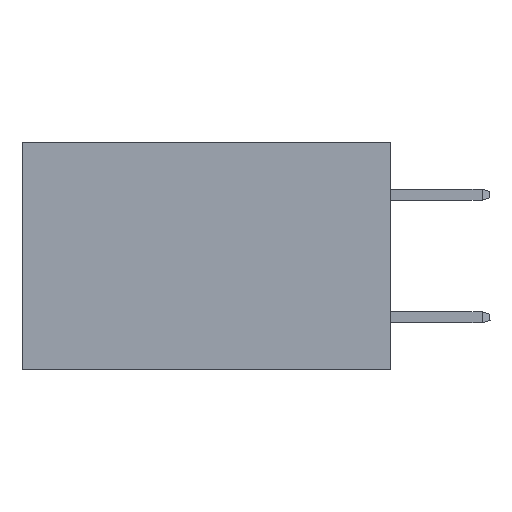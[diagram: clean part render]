
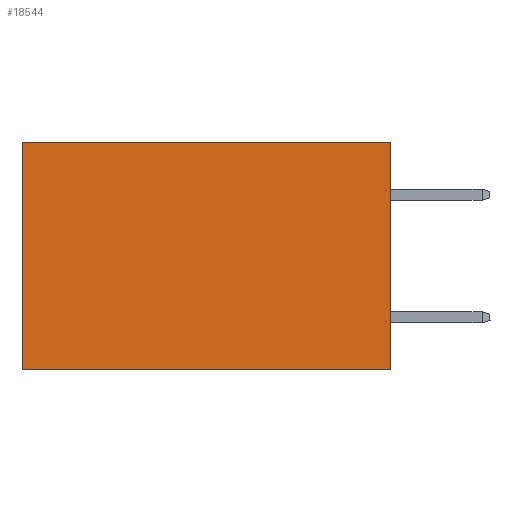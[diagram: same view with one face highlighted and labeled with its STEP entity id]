
A CAD part, left-side view. The second image highlights one B-rep face of the part: STEP entity #18544.
In plain terms, the highlighted planar face has unit normal (-1, 0, 0).
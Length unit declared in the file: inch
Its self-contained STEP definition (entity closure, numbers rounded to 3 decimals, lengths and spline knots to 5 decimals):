
#180 = VERTEX_POINT ( 'NONE', #13784 ) ;
#320 = VECTOR ( 'NONE', #20988, 39.37008 ) ;
#713 = EDGE_CURVE ( 'NONE', #6333, #1933, #5718, .T. ) ;
#1468 = DIRECTION ( 'NONE',  ( 1., 0., 0. ) ) ;
#1933 = VERTEX_POINT ( 'NONE', #5742 ) ;
#2020 = CARTESIAN_POINT ( 'NONE',  ( 0.2875, 0.6, 0. ) ) ;
#3017 = ORIENTED_EDGE ( 'NONE', *, *, #713, .F. ) ;
#4974 = CARTESIAN_POINT ( 'NONE',  ( 0.2875, 0., 0. ) ) ;
#5698 = ORIENTED_EDGE ( 'NONE', *, *, #15745, .T. ) ;
#5718 = LINE ( 'NONE', #10823, #8137 ) ;
#5742 = CARTESIAN_POINT ( 'NONE',  ( 0.2875, 0.6, -0.37 ) ) ;
#6333 = VERTEX_POINT ( 'NONE', #21174 ) ;
#7800 = DIRECTION ( 'NONE',  ( 0., 1., 0. ) ) ;
#8123 = PLANE ( 'NONE',  #17320 ) ;
#8137 = VECTOR ( 'NONE', #14182, 39.37008 ) ;
#8636 = LINE ( 'NONE', #2020, #320 ) ;
#10090 = CARTESIAN_POINT ( 'NONE',  ( 0.2875, 0., 0. ) ) ;
#10389 = ORIENTED_EDGE ( 'NONE', *, *, #11664, .T. ) ;
#10823 = CARTESIAN_POINT ( 'NONE',  ( 0.2875, 0., -0.37 ) ) ;
#11453 = VERTEX_POINT ( 'NONE', #13164 ) ;
#11664 = EDGE_CURVE ( 'NONE', #180, #1933, #8636, .T. ) ;
#11949 = DIRECTION ( 'NONE',  ( 0., 0., -1. ) ) ;
#12120 = EDGE_LOOP ( 'NONE', ( #10389, #3017, #12551, #5698 ) ) ;
#12551 = ORIENTED_EDGE ( 'NONE', *, *, #20283, .F. ) ;
#12940 = CARTESIAN_POINT ( 'NONE',  ( 0.2875, 0., 0. ) ) ;
#13164 = CARTESIAN_POINT ( 'NONE',  ( 0.2875, 0., 0. ) ) ;
#13668 = LINE ( 'NONE', #12940, #14219 ) ;
#13784 = CARTESIAN_POINT ( 'NONE',  ( 0.2875, 0.6, 0. ) ) ;
#14182 = DIRECTION ( 'NONE',  ( 0., 1., 0. ) ) ;
#14219 = VECTOR ( 'NONE', #7800, 39.37008 ) ;
#15089 = DIRECTION ( 'NONE',  ( 0., 0., -1. ) ) ;
#15745 = EDGE_CURVE ( 'NONE', #11453, #180, #13668, .T. ) ;
#17320 = AXIS2_PLACEMENT_3D ( 'NONE', #4974, #1468, #15089 ) ;
#18544 = ADVANCED_FACE ( 'NONE', ( #21994 ), #8123, .F. ) ;
#19860 = VECTOR ( 'NONE', #11949, 39.37008 ) ;
#20283 = EDGE_CURVE ( 'NONE', #11453, #6333, #21502, .T. ) ;
#20988 = DIRECTION ( 'NONE',  ( 0., 0., -1. ) ) ;
#21174 = CARTESIAN_POINT ( 'NONE',  ( 0.2875, 0., -0.37 ) ) ;
#21502 = LINE ( 'NONE', #10090, #19860 ) ;
#21994 = FACE_OUTER_BOUND ( 'NONE', #12120, .T. ) ;
